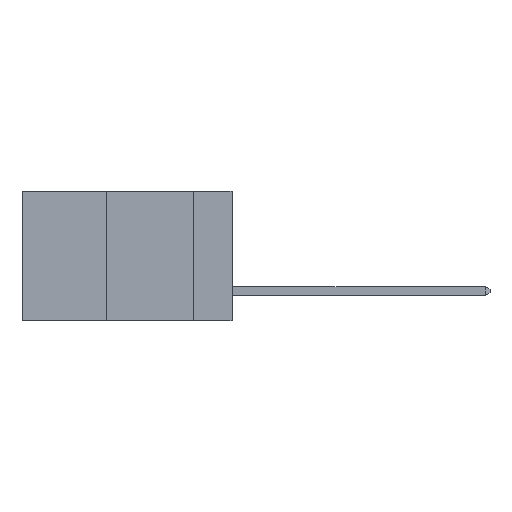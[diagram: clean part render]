
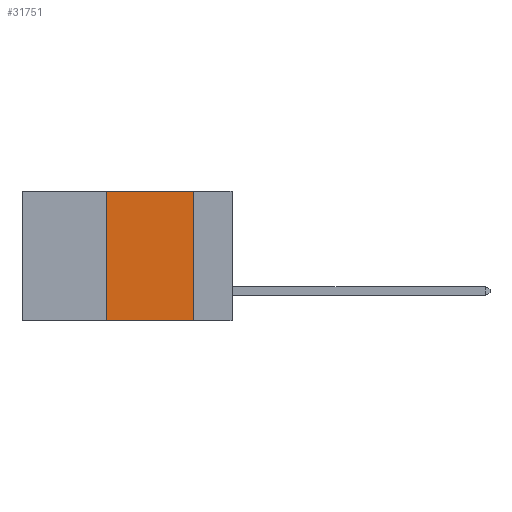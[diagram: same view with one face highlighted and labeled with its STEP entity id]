
A CAD part, left-side view. The second image highlights one B-rep face of the part: STEP entity #31751.
In plain terms, the highlighted planar face has unit normal (-1, 0, 0).
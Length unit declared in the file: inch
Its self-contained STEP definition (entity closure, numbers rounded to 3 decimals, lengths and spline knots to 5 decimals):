
#1114 = DIRECTION ( 'NONE',  ( 0., 0., 1. ) ) ;
#1665 = VERTEX_POINT ( 'NONE', #33616 ) ;
#3768 = CARTESIAN_POINT ( 'NONE',  ( 0., 0.36, -0.37 ) ) ;
#5266 = ORIENTED_EDGE ( 'NONE', *, *, #25207, .T. ) ;
#5331 = VECTOR ( 'NONE', #1114, 39.37008 ) ;
#5974 = CARTESIAN_POINT ( 'NONE',  ( 0., 0.6, 0. ) ) ;
#6126 = CARTESIAN_POINT ( 'NONE',  ( 0., 0.11, 0. ) ) ;
#8541 = PLANE ( 'NONE',  #25152 ) ;
#9354 = EDGE_CURVE ( 'NONE', #1665, #11314, #26239, .T. ) ;
#10790 = ORIENTED_EDGE ( 'NONE', *, *, #12702, .F. ) ;
#10941 = LINE ( 'NONE', #23300, #17009 ) ;
#11136 = DIRECTION ( 'NONE',  ( 1., 0., 0. ) ) ;
#11314 = VERTEX_POINT ( 'NONE', #24671 ) ;
#12345 = VECTOR ( 'NONE', #29507, 39.37008 ) ;
#12702 = EDGE_CURVE ( 'NONE', #11314, #33224, #26806, .T. ) ;
#13644 = CARTESIAN_POINT ( 'NONE',  ( 0., 0.6, 0. ) ) ;
#13950 = VERTEX_POINT ( 'NONE', #3768 ) ;
#15822 = CARTESIAN_POINT ( 'NONE',  ( 0., 0.11, -0.37 ) ) ;
#17009 = VECTOR ( 'NONE', #25968, 39.37008 ) ;
#22541 = ORIENTED_EDGE ( 'NONE', *, *, #9354, .F. ) ;
#22916 = ORIENTED_EDGE ( 'NONE', *, *, #30058, .F. ) ;
#23300 = CARTESIAN_POINT ( 'NONE',  ( 0., 0.6, -0.37 ) ) ;
#24347 = DIRECTION ( 'NONE',  ( 0., 0., -1. ) ) ;
#24671 = CARTESIAN_POINT ( 'NONE',  ( 0., 0.11, 0. ) ) ;
#25152 = AXIS2_PLACEMENT_3D ( 'NONE', #13644, #11136, #29439 ) ;
#25207 = EDGE_CURVE ( 'NONE', #13950, #33224, #10941, .T. ) ;
#25446 = EDGE_LOOP ( 'NONE', ( #10790, #22541, #22916, #5266 ) ) ;
#25968 = DIRECTION ( 'NONE',  ( 0., -1., 0. ) ) ;
#26146 = LINE ( 'NONE', #27228, #5331 ) ;
#26239 = LINE ( 'NONE', #5974, #12345 ) ;
#26806 = LINE ( 'NONE', #6126, #33780 ) ;
#27228 = CARTESIAN_POINT ( 'NONE',  ( 0., 0.36, 0. ) ) ;
#29439 = DIRECTION ( 'NONE',  ( 0., 0., -1. ) ) ;
#29507 = DIRECTION ( 'NONE',  ( 0., -1., 0. ) ) ;
#30058 = EDGE_CURVE ( 'NONE', #13950, #1665, #26146, .T. ) ;
#31751 = ADVANCED_FACE ( 'NONE', ( #33868 ), #8541, .F. ) ;
#33224 = VERTEX_POINT ( 'NONE', #15822 ) ;
#33616 = CARTESIAN_POINT ( 'NONE',  ( 0., 0.36, 0. ) ) ;
#33780 = VECTOR ( 'NONE', #24347, 39.37008 ) ;
#33868 = FACE_OUTER_BOUND ( 'NONE', #25446, .T. ) ;
